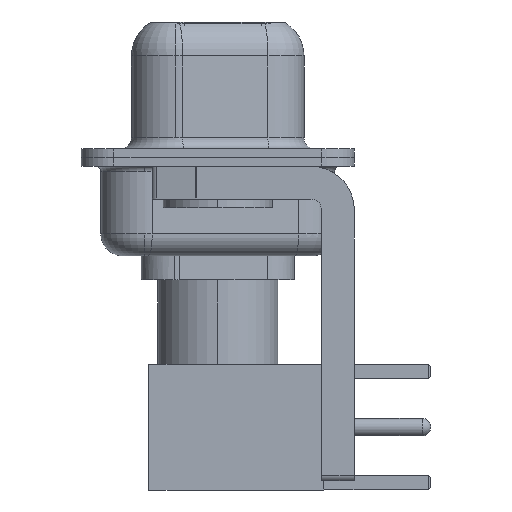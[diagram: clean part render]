
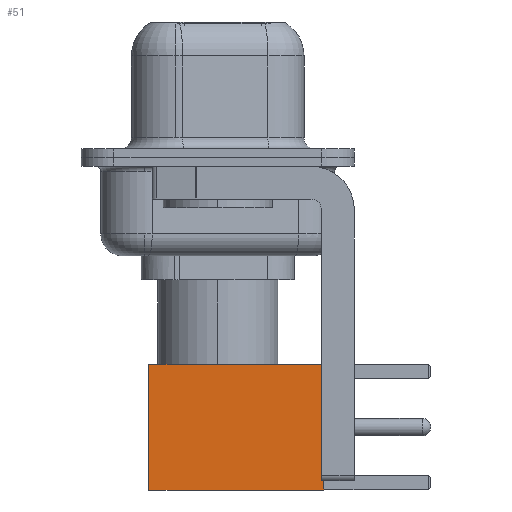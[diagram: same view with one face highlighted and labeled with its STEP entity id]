
A CAD part, left-side view. The second image highlights one B-rep face of the part: STEP entity #51.
In plain terms, the highlighted face is planar.
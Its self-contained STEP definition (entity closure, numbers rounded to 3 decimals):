
#51 = ADVANCED_FACE ( 'NONE', ( #10559 ), #5221, .T. ) ;
#195 = VECTOR ( 'NONE', #6688, 1000. ) ;
#205 = EDGE_LOOP ( 'NONE', ( #7260, #8006, #7359, #5560 ) ) ;
#311 = DIRECTION ( 'NONE',  ( -1., 0., 0. ) ) ;
#319 = CARTESIAN_POINT ( 'NONE',  ( 2.875, 2.875, 0. ) ) ;
#1379 = VECTOR ( 'NONE', #14028, 1000. ) ;
#1459 = VERTEX_POINT ( 'NONE', #13444 ) ;
#2913 = CARTESIAN_POINT ( 'NONE',  ( -2.875, 2.875, 8. ) ) ;
#3331 = LINE ( 'NONE', #12294, #8442 ) ;
#3859 = VERTEX_POINT ( 'NONE', #2913 ) ;
#3903 = DIRECTION ( 'NONE',  ( 0., 1., 0. ) ) ;
#5221 = PLANE ( 'NONE',  #12883 ) ;
#5439 = EDGE_CURVE ( 'NONE', #10025, #3859, #15517, .T. ) ;
#5560 = ORIENTED_EDGE ( 'NONE', *, *, #5439, .F. ) ;
#5892 = DIRECTION ( 'NONE',  ( 0., 0., -1. ) ) ;
#6688 = DIRECTION ( 'NONE',  ( -1., 0., 0. ) ) ;
#7260 = ORIENTED_EDGE ( 'NONE', *, *, #13570, .T. ) ;
#7359 = ORIENTED_EDGE ( 'NONE', *, *, #12458, .F. ) ;
#7681 = CARTESIAN_POINT ( 'NONE',  ( 2.875, 2.875, 0. ) ) ;
#7908 = CARTESIAN_POINT ( 'NONE',  ( 0., 2.875, 0. ) ) ;
#8006 = ORIENTED_EDGE ( 'NONE', *, *, #8266, .T. ) ;
#8266 = EDGE_CURVE ( 'NONE', #12574, #1459, #9151, .T. ) ;
#8442 = VECTOR ( 'NONE', #5892, 1000. ) ;
#9151 = LINE ( 'NONE', #7908, #195 ) ;
#10025 = VERTEX_POINT ( 'NONE', #10812 ) ;
#10559 = FACE_OUTER_BOUND ( 'NONE', #205, .T. ) ;
#10812 = CARTESIAN_POINT ( 'NONE',  ( 2.875, 2.875, 8. ) ) ;
#11544 = DIRECTION ( 'NONE',  ( 0., 0., 1. ) ) ;
#11629 = LINE ( 'NONE', #319, #1379 ) ;
#12294 = CARTESIAN_POINT ( 'NONE',  ( -2.875, 2.875, 0. ) ) ;
#12458 = EDGE_CURVE ( 'NONE', #3859, #1459, #3331, .T. ) ;
#12574 = VERTEX_POINT ( 'NONE', #7681 ) ;
#12883 = AXIS2_PLACEMENT_3D ( 'NONE', #14187, #3903, #11544 ) ;
#13444 = CARTESIAN_POINT ( 'NONE',  ( -2.875, 2.875, 0. ) ) ;
#13570 = EDGE_CURVE ( 'NONE', #10025, #12574, #11629, .T. ) ;
#13934 = CARTESIAN_POINT ( 'NONE',  ( 0., 2.875, 8. ) ) ;
#14028 = DIRECTION ( 'NONE',  ( 0., 0., -1. ) ) ;
#14187 = CARTESIAN_POINT ( 'NONE',  ( 2.875, 2.875, 0. ) ) ;
#14905 = VECTOR ( 'NONE', #311, 1000. ) ;
#15517 = LINE ( 'NONE', #13934, #14905 ) ;
